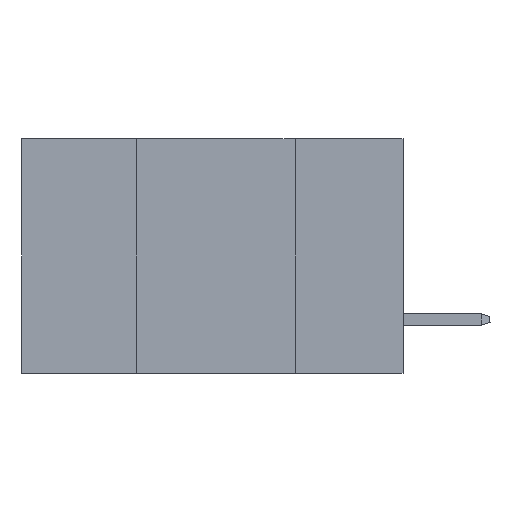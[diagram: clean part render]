
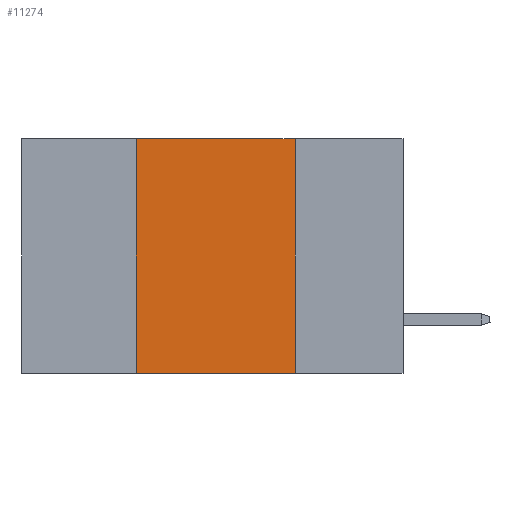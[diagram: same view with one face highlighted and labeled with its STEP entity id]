
A CAD part, left-side view. The second image highlights one B-rep face of the part: STEP entity #11274.
In plain terms, the highlighted planar face has unit normal (-1, 0, 0).
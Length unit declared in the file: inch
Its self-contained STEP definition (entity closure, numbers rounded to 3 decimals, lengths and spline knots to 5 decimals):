
#970 = EDGE_CURVE ( 'NONE', #4694, #1450, #5748, .T. ) ;
#1450 = VERTEX_POINT ( 'NONE', #17389 ) ;
#1739 = ORIENTED_EDGE ( 'NONE', *, *, #970, .T. ) ;
#2129 = VECTOR ( 'NONE', #10719, 39.37008 ) ;
#3774 = EDGE_CURVE ( 'NONE', #20093, #14888, #14729, .T. ) ;
#4173 = CARTESIAN_POINT ( 'NONE',  ( 0., 0.17, 0. ) ) ;
#4694 = VERTEX_POINT ( 'NONE', #6747 ) ;
#4999 = VECTOR ( 'NONE', #20788, 39.37008 ) ;
#5748 = LINE ( 'NONE', #12346, #2129 ) ;
#6331 = CARTESIAN_POINT ( 'NONE',  ( 0., 0.42, 0. ) ) ;
#6720 = DIRECTION ( 'NONE',  ( 0., -1., 0. ) ) ;
#6747 = CARTESIAN_POINT ( 'NONE',  ( 0., 0.42, -0.37 ) ) ;
#7739 = PLANE ( 'NONE',  #11101 ) ;
#7746 = EDGE_CURVE ( 'NONE', #14888, #1450, #17455, .T. ) ;
#7754 = ORIENTED_EDGE ( 'NONE', *, *, #7746, .F. ) ;
#9467 = CARTESIAN_POINT ( 'NONE',  ( 0., 0.6, 0. ) ) ;
#9818 = DIRECTION ( 'NONE',  ( 0., 0., 1. ) ) ;
#10579 = EDGE_CURVE ( 'NONE', #4694, #20093, #18244, .T. ) ;
#10719 = DIRECTION ( 'NONE',  ( 0., -1., 0. ) ) ;
#11101 = AXIS2_PLACEMENT_3D ( 'NONE', #9467, #17476, #20704 ) ;
#11274 = ADVANCED_FACE ( 'NONE', ( #21018 ), #7739, .F. ) ;
#11812 = VECTOR ( 'NONE', #9818, 39.37008 ) ;
#11891 = CARTESIAN_POINT ( 'NONE',  ( 0., 0.42, 0. ) ) ;
#12346 = CARTESIAN_POINT ( 'NONE',  ( 0., 0.6, -0.37 ) ) ;
#13319 = CARTESIAN_POINT ( 'NONE',  ( 0., 0.6, 0. ) ) ;
#14041 = EDGE_LOOP ( 'NONE', ( #7754, #15849, #19588, #1739 ) ) ;
#14729 = LINE ( 'NONE', #13319, #15634 ) ;
#14888 = VERTEX_POINT ( 'NONE', #20453 ) ;
#15634 = VECTOR ( 'NONE', #6720, 39.37008 ) ;
#15849 = ORIENTED_EDGE ( 'NONE', *, *, #3774, .F. ) ;
#17389 = CARTESIAN_POINT ( 'NONE',  ( 0., 0.17, -0.37 ) ) ;
#17455 = LINE ( 'NONE', #4173, #4999 ) ;
#17476 = DIRECTION ( 'NONE',  ( 1., 0., 0. ) ) ;
#18244 = LINE ( 'NONE', #11891, #11812 ) ;
#19588 = ORIENTED_EDGE ( 'NONE', *, *, #10579, .F. ) ;
#20093 = VERTEX_POINT ( 'NONE', #6331 ) ;
#20453 = CARTESIAN_POINT ( 'NONE',  ( 0., 0.17, 0. ) ) ;
#20704 = DIRECTION ( 'NONE',  ( 0., 0., -1. ) ) ;
#20788 = DIRECTION ( 'NONE',  ( 0., 0., -1. ) ) ;
#21018 = FACE_OUTER_BOUND ( 'NONE', #14041, .T. ) ;
